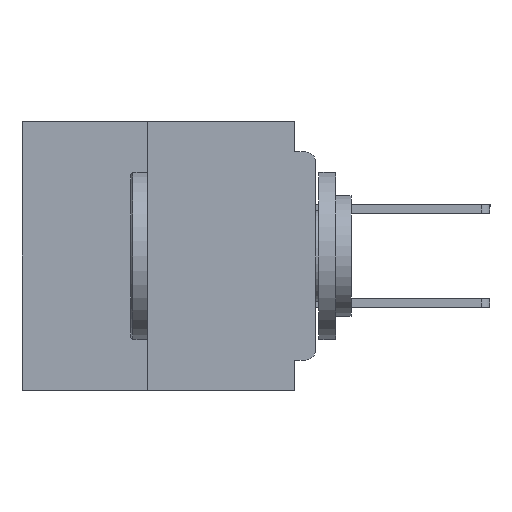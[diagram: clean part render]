
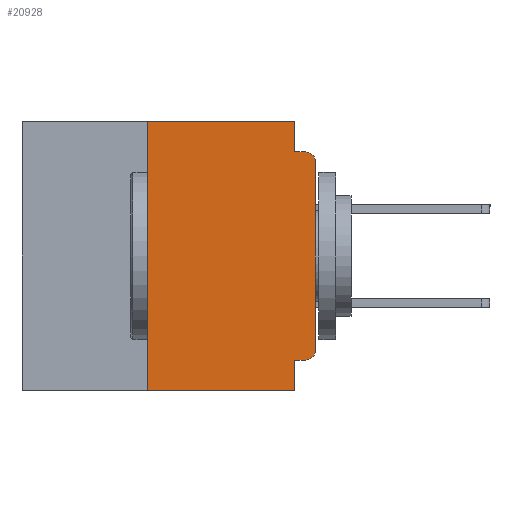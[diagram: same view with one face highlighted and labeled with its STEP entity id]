
A CAD part, left-side view. The second image highlights one B-rep face of the part: STEP entity #20928.
In plain terms, the highlighted planar face has unit normal (-1, 0, 0).
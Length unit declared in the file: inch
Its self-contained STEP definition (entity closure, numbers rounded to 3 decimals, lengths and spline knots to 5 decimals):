
#265 = LINE ( 'NONE', #16955, #19197 ) ;
#1659 = CARTESIAN_POINT ( 'NONE',  ( 0., 0.437, -0.4 ) ) ;
#1702 = EDGE_CURVE ( 'NONE', #10775, #32757, #37332, .T. ) ;
#2323 = EDGE_CURVE ( 'NONE', #34857, #14360, #265, .T. ) ;
#3248 = VERTEX_POINT ( 'NONE', #18731 ) ;
#3809 = VECTOR ( 'NONE', #17515, 39.37008 ) ;
#4788 = CARTESIAN_POINT ( 'NONE',  ( 0., 0.25, -0.4 ) ) ;
#4945 = LINE ( 'NONE', #4788, #43640 ) ;
#5537 = DIRECTION ( 'NONE',  ( 0., -1., 0. ) ) ;
#5623 = LINE ( 'NONE', #39354, #24395 ) ;
#5846 = CARTESIAN_POINT ( 'NONE',  ( 0., 0., -0.34 ) ) ;
#9125 = LINE ( 'NONE', #29192, #46605 ) ;
#10622 = DIRECTION ( 'NONE',  ( 0., -1., 0. ) ) ;
#10687 = EDGE_LOOP ( 'NONE', ( #24711, #21575, #14471, #42009, #20497, #48590, #28141, #29692, #33190, #47412 ) ) ;
#10775 = VERTEX_POINT ( 'NONE', #46634 ) ;
#11056 = EDGE_CURVE ( 'NONE', #14360, #47753, #18080, .T. ) ;
#11334 = CARTESIAN_POINT ( 'NONE',  ( 0., 0., -0.06 ) ) ;
#12821 = EDGE_CURVE ( 'NONE', #28088, #20888, #9125, .T. ) ;
#14133 = CARTESIAN_POINT ( 'NONE',  ( 0., 0.031, -0.4 ) ) ;
#14360 = VERTEX_POINT ( 'NONE', #11334 ) ;
#14471 = ORIENTED_EDGE ( 'NONE', *, *, #32048, .F. ) ;
#14568 = DIRECTION ( 'NONE',  ( 0., 0., 1. ) ) ;
#14651 = EDGE_CURVE ( 'NONE', #32443, #32757, #35871, .T. ) ;
#15405 = CIRCLE ( 'NONE', #44405, 0.015 ) ;
#15532 = CARTESIAN_POINT ( 'NONE',  ( 0., 0.015, -0.06 ) ) ;
#15955 = DIRECTION ( 'NONE',  ( -1., 0., 0. ) ) ;
#16189 = DIRECTION ( 'NONE',  ( 0., 0., 1. ) ) ;
#16955 = CARTESIAN_POINT ( 'NONE',  ( 0., 0., 0. ) ) ;
#17183 = CARTESIAN_POINT ( 'NONE',  ( 0., 0.031, 0. ) ) ;
#17515 = DIRECTION ( 'NONE',  ( 0., 1., 0. ) ) ;
#18080 = CIRCLE ( 'NONE', #38773, 0.015 ) ;
#18731 = CARTESIAN_POINT ( 'NONE',  ( 0., 0.031, -0.045 ) ) ;
#19197 = VECTOR ( 'NONE', #14568, 39.37008 ) ;
#19281 = DIRECTION ( 'NONE',  ( 0., 0., -1. ) ) ;
#19682 = LINE ( 'NONE', #23635, #38334 ) ;
#20497 = ORIENTED_EDGE ( 'NONE', *, *, #12821, .F. ) ;
#20888 = VERTEX_POINT ( 'NONE', #17183 ) ;
#20912 = EDGE_CURVE ( 'NONE', #38404, #10775, #33654, .T. ) ;
#20928 = ADVANCED_FACE ( 'NONE', ( #42504 ), #43671, .F. ) ;
#21315 = EDGE_CURVE ( 'NONE', #32443, #28088, #4945, .T. ) ;
#21575 = ORIENTED_EDGE ( 'NONE', *, *, #11056, .T. ) ;
#23635 = CARTESIAN_POINT ( 'NONE',  ( 0., 0., -0.045 ) ) ;
#24075 = CARTESIAN_POINT ( 'NONE',  ( 0., 0.031, -0.4 ) ) ;
#24395 = VECTOR ( 'NONE', #43149, 39.37008 ) ;
#24711 = ORIENTED_EDGE ( 'NONE', *, *, #2323, .T. ) ;
#25025 = DIRECTION ( 'NONE',  ( 0., 0., -1. ) ) ;
#27343 = DIRECTION ( 'NONE',  ( 0., -1., 0. ) ) ;
#27376 = VECTOR ( 'NONE', #32588, 39.37008 ) ;
#28088 = VERTEX_POINT ( 'NONE', #29040 ) ;
#28141 = ORIENTED_EDGE ( 'NONE', *, *, #14651, .T. ) ;
#28559 = CARTESIAN_POINT ( 'NONE',  ( 0., 0.437, 0. ) ) ;
#29040 = CARTESIAN_POINT ( 'NONE',  ( 0., 0.25, 0. ) ) ;
#29192 = CARTESIAN_POINT ( 'NONE',  ( 0., 0.437, 0. ) ) ;
#29692 = ORIENTED_EDGE ( 'NONE', *, *, #1702, .F. ) ;
#31492 = EDGE_CURVE ( 'NONE', #20888, #3248, #5623, .T. ) ;
#32048 = EDGE_CURVE ( 'NONE', #3248, #47753, #19682, .T. ) ;
#32443 = VERTEX_POINT ( 'NONE', #44726 ) ;
#32588 = DIRECTION ( 'NONE',  ( 0., 0., -1. ) ) ;
#32757 = VERTEX_POINT ( 'NONE', #24075 ) ;
#33190 = ORIENTED_EDGE ( 'NONE', *, *, #20912, .F. ) ;
#33654 = LINE ( 'NONE', #36090, #3809 ) ;
#34686 = VECTOR ( 'NONE', #5537, 39.37008 ) ;
#34857 = VERTEX_POINT ( 'NONE', #5846 ) ;
#35871 = LINE ( 'NONE', #1659, #34686 ) ;
#36090 = CARTESIAN_POINT ( 'NONE',  ( 0., 0., -0.355 ) ) ;
#36571 = EDGE_CURVE ( 'NONE', #38404, #34857, #15405, .T. ) ;
#37332 = LINE ( 'NONE', #14133, #27376 ) ;
#38281 = CARTESIAN_POINT ( 'NONE',  ( 0., 0.015, -0.34 ) ) ;
#38334 = VECTOR ( 'NONE', #27343, 39.37008 ) ;
#38404 = VERTEX_POINT ( 'NONE', #42087 ) ;
#38773 = AXIS2_PLACEMENT_3D ( 'NONE', #15532, #41657, #19281 ) ;
#39354 = CARTESIAN_POINT ( 'NONE',  ( 0., 0.031, 0. ) ) ;
#41312 = AXIS2_PLACEMENT_3D ( 'NONE', #28559, #47440, #25025 ) ;
#41657 = DIRECTION ( 'NONE',  ( -1., 0., 0. ) ) ;
#42009 = ORIENTED_EDGE ( 'NONE', *, *, #31492, .F. ) ;
#42077 = DIRECTION ( 'NONE',  ( 0., 0., -1. ) ) ;
#42087 = CARTESIAN_POINT ( 'NONE',  ( 0., 0.015, -0.355 ) ) ;
#42504 = FACE_OUTER_BOUND ( 'NONE', #10687, .T. ) ;
#42627 = CARTESIAN_POINT ( 'NONE',  ( 0., 0.015, -0.045 ) ) ;
#43149 = DIRECTION ( 'NONE',  ( 0., 0., -1. ) ) ;
#43640 = VECTOR ( 'NONE', #16189, 39.37008 ) ;
#43671 = PLANE ( 'NONE',  #41312 ) ;
#44405 = AXIS2_PLACEMENT_3D ( 'NONE', #38281, #15955, #42077 ) ;
#44726 = CARTESIAN_POINT ( 'NONE',  ( 0., 0.25, -0.4 ) ) ;
#46605 = VECTOR ( 'NONE', #10622, 39.37008 ) ;
#46634 = CARTESIAN_POINT ( 'NONE',  ( 0., 0.031, -0.355 ) ) ;
#47412 = ORIENTED_EDGE ( 'NONE', *, *, #36571, .T. ) ;
#47440 = DIRECTION ( 'NONE',  ( 1., 0., 0. ) ) ;
#47753 = VERTEX_POINT ( 'NONE', #42627 ) ;
#48590 = ORIENTED_EDGE ( 'NONE', *, *, #21315, .F. ) ;
